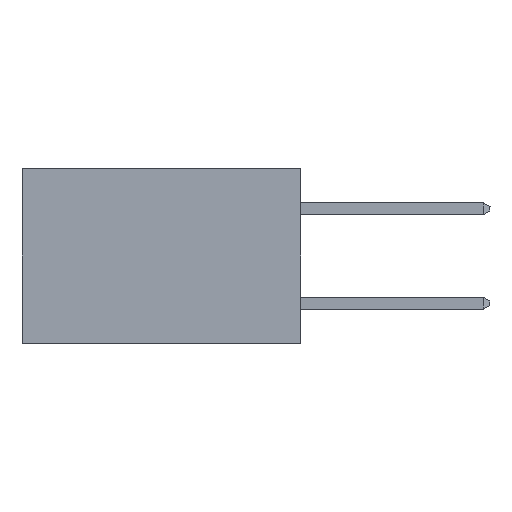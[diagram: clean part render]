
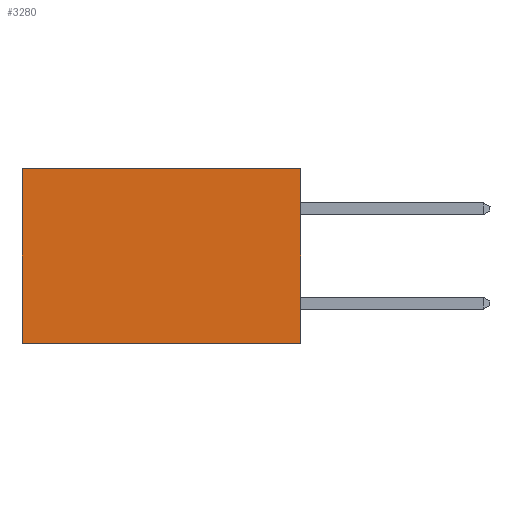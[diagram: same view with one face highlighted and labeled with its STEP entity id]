
A CAD part, left-side view. The second image highlights one B-rep face of the part: STEP entity #3280.
In plain terms, the highlighted planar face has unit normal (-1, 0, 0).
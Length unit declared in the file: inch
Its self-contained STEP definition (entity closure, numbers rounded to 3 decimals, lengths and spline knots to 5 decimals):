
#12 = CARTESIAN_POINT ( 'NONE',  ( 0.277, 0., -0.37 ) ) ;
#130 = DIRECTION ( 'NONE',  ( 0., 0., -1. ) ) ;
#636 = VERTEX_POINT ( 'NONE', #3029 ) ;
#700 = PLANE ( 'NONE',  #3276 ) ;
#777 = DIRECTION ( 'NONE',  ( 1., 0., 0. ) ) ;
#851 = ORIENTED_EDGE ( 'NONE', *, *, #8737, .T. ) ;
#863 = EDGE_CURVE ( 'NONE', #2379, #636, #8843, .T. ) ;
#907 = ORIENTED_EDGE ( 'NONE', *, *, #863, .F. ) ;
#972 = ORIENTED_EDGE ( 'NONE', *, *, #8984, .T. ) ;
#1121 = CARTESIAN_POINT ( 'NONE',  ( 0.277, 0., -0.37 ) ) ;
#1340 = ORIENTED_EDGE ( 'NONE', *, *, #6217, .F. ) ;
#1535 = VERTEX_POINT ( 'NONE', #5385 ) ;
#1751 = VERTEX_POINT ( 'NONE', #6932 ) ;
#1841 = FACE_OUTER_BOUND ( 'NONE', #6849, .T. ) ;
#1845 = CARTESIAN_POINT ( 'NONE',  ( 0.277, 0., 0. ) ) ;
#1903 = VECTOR ( 'NONE', #6976, 39.37008 ) ;
#2020 = VECTOR ( 'NONE', #7397, 39.37008 ) ;
#2110 = LINE ( 'NONE', #12, #3863 ) ;
#2343 = CARTESIAN_POINT ( 'NONE',  ( 0.277, 0., -0.37 ) ) ;
#2379 = VERTEX_POINT ( 'NONE', #1121 ) ;
#3023 = DIRECTION ( 'NONE',  ( 0., 1., 0. ) ) ;
#3029 = CARTESIAN_POINT ( 'NONE',  ( 0.277, 0.59, -0.37 ) ) ;
#3062 = CARTESIAN_POINT ( 'NONE',  ( 0.277, 0.59, -0.37 ) ) ;
#3276 = AXIS2_PLACEMENT_3D ( 'NONE', #2343, #777, #3373 ) ;
#3280 = ADVANCED_FACE ( 'NONE', ( #1841 ), #700, .F. ) ;
#3373 = DIRECTION ( 'NONE',  ( 0., 0., -1. ) ) ;
#3863 = VECTOR ( 'NONE', #130, 39.37008 ) ;
#5385 = CARTESIAN_POINT ( 'NONE',  ( 0.277, 0.59, 0. ) ) ;
#5565 = CARTESIAN_POINT ( 'NONE',  ( 0.277, 0., -0.37 ) ) ;
#5910 = LINE ( 'NONE', #1845, #1903 ) ;
#6217 = EDGE_CURVE ( 'NONE', #1751, #2379, #2110, .T. ) ;
#6225 = LINE ( 'NONE', #3062, #2020 ) ;
#6849 = EDGE_LOOP ( 'NONE', ( #851, #907, #1340, #972 ) ) ;
#6932 = CARTESIAN_POINT ( 'NONE',  ( 0.277, 0., 0. ) ) ;
#6976 = DIRECTION ( 'NONE',  ( 0., 1., 0. ) ) ;
#7397 = DIRECTION ( 'NONE',  ( 0., 0., -1. ) ) ;
#8660 = VECTOR ( 'NONE', #3023, 39.37008 ) ;
#8737 = EDGE_CURVE ( 'NONE', #1535, #636, #6225, .T. ) ;
#8843 = LINE ( 'NONE', #5565, #8660 ) ;
#8984 = EDGE_CURVE ( 'NONE', #1751, #1535, #5910, .T. ) ;
